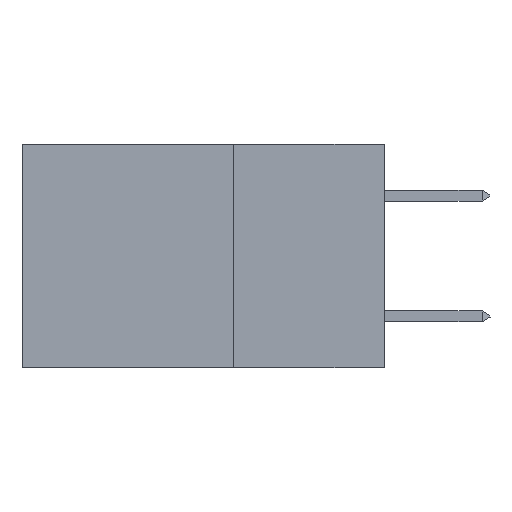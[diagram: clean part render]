
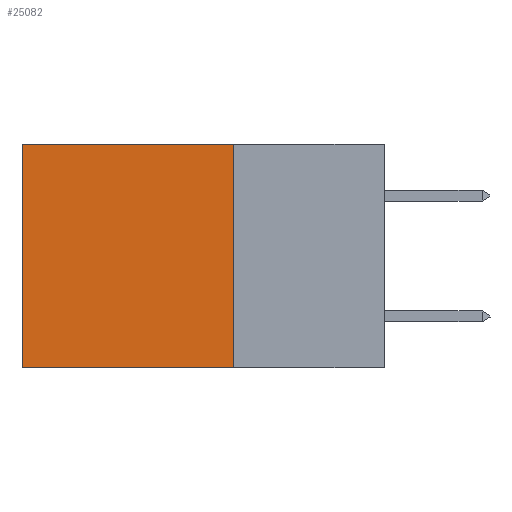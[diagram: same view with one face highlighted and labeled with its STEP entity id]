
A CAD part, left-side view. The second image highlights one B-rep face of the part: STEP entity #25082.
In plain terms, the highlighted planar face has unit normal (-1, 0, 0).
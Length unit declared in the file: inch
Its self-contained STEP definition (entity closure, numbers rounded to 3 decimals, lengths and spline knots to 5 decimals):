
#662 = CARTESIAN_POINT ( 'NONE',  ( 0.2875, 0.25, -0.37 ) ) ;
#1352 = LINE ( 'NONE', #10927, #15501 ) ;
#2765 = DIRECTION ( 'NONE',  ( 0., 0., -1. ) ) ;
#3963 = LINE ( 'NONE', #19161, #27682 ) ;
#5248 = EDGE_CURVE ( 'NONE', #22536, #6643, #1352, .T. ) ;
#5513 = ORIENTED_EDGE ( 'NONE', *, *, #20342, .T. ) ;
#6532 = LINE ( 'NONE', #19793, #31077 ) ;
#6643 = VERTEX_POINT ( 'NONE', #30880 ) ;
#7268 = DIRECTION ( 'NONE',  ( 0., 0., -1. ) ) ;
#7451 = DIRECTION ( 'NONE',  ( 0., 1., 0. ) ) ;
#9195 = ORIENTED_EDGE ( 'NONE', *, *, #33741, .F. ) ;
#10927 = CARTESIAN_POINT ( 'NONE',  ( 0.2875, 0.6, 0. ) ) ;
#12017 = AXIS2_PLACEMENT_3D ( 'NONE', #31978, #34721, #7268 ) ;
#12635 = PLANE ( 'NONE',  #12017 ) ;
#15501 = VECTOR ( 'NONE', #2765, 39.37008 ) ;
#16730 = DIRECTION ( 'NONE',  ( 0., 0., -1. ) ) ;
#18574 = LINE ( 'NONE', #35325, #22460 ) ;
#18932 = CARTESIAN_POINT ( 'NONE',  ( 0.2875, 0.25, 0. ) ) ;
#19161 = CARTESIAN_POINT ( 'NONE',  ( 0.2875, 0.25, 0. ) ) ;
#19793 = CARTESIAN_POINT ( 'NONE',  ( 0.2875, 0.25, 0. ) ) ;
#20342 = EDGE_CURVE ( 'NONE', #29357, #22536, #3963, .T. ) ;
#21347 = CARTESIAN_POINT ( 'NONE',  ( 0.2875, 0.6, 0. ) ) ;
#21419 = ORIENTED_EDGE ( 'NONE', *, *, #5248, .T. ) ;
#22460 = VECTOR ( 'NONE', #29793, 39.37008 ) ;
#22536 = VERTEX_POINT ( 'NONE', #21347 ) ;
#23928 = FACE_OUTER_BOUND ( 'NONE', #27515, .T. ) ;
#25082 = ADVANCED_FACE ( 'NONE', ( #23928 ), #12635, .F. ) ;
#26637 = EDGE_CURVE ( 'NONE', #29357, #30580, #6532, .T. ) ;
#27515 = EDGE_LOOP ( 'NONE', ( #21419, #9195, #29652, #5513 ) ) ;
#27682 = VECTOR ( 'NONE', #7451, 39.37008 ) ;
#29357 = VERTEX_POINT ( 'NONE', #18932 ) ;
#29652 = ORIENTED_EDGE ( 'NONE', *, *, #26637, .F. ) ;
#29793 = DIRECTION ( 'NONE',  ( 0., 1., 0. ) ) ;
#30580 = VERTEX_POINT ( 'NONE', #662 ) ;
#30880 = CARTESIAN_POINT ( 'NONE',  ( 0.2875, 0.6, -0.37 ) ) ;
#31077 = VECTOR ( 'NONE', #16730, 39.37008 ) ;
#31978 = CARTESIAN_POINT ( 'NONE',  ( 0.2875, 0.25, 0. ) ) ;
#33741 = EDGE_CURVE ( 'NONE', #30580, #6643, #18574, .T. ) ;
#34721 = DIRECTION ( 'NONE',  ( 1., 0., 0. ) ) ;
#35325 = CARTESIAN_POINT ( 'NONE',  ( 0.2875, 0.25, -0.37 ) ) ;
